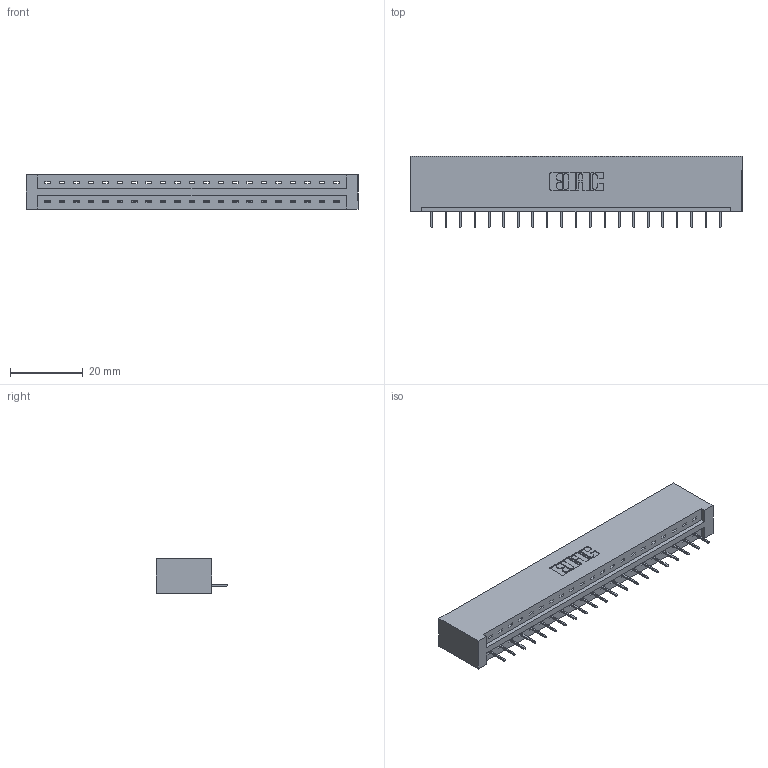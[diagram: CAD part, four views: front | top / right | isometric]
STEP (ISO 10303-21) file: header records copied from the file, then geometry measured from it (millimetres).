
FILE_DESCRIPTION (( 'STEP AP203' ), '1' );
FILE_NAME ('387-021-524-101.STEP', '2019-10-02T23:44:25', ( '' ), ( '' ), 'SwSTEP 2.0', 'SolidWorks 2016', '' );
FILE_SCHEMA (( 'CONFIG_CONTROL_DESIGN' ));
Length unit declared in the file: inch
Products named in the file (3): 387-021-524-101; 337 Part_No Mounting Lugs; 345-292-001_345-293-124
Assembly tree (22 placements, depth 2):
  387-021-524-101
    337 Part_No Mounting Lugs
    345-292-001_345-293-124  x21
Bounding box: 91.08 x 19.69 x 9.4 mm (x, y, z)
Volume: 9859.7 mm3; surface area: 9761.7 mm2
Topology: 22 solids, 22 shells, 1492 faces, 4319 edges, 2794 vertices
Faces by surface type: plane 1158, cylinder 334
Entity records: 18123 total; most frequent: CARTESIAN_POINT 3161, ORIENTED_EDGE 3118, DIRECTION 2697, EDGE_CURVE 1559, LINE 1443, VECTOR 1443, VERTEX_POINT 1034, AXIS2_PLACEMENT_3D 627
